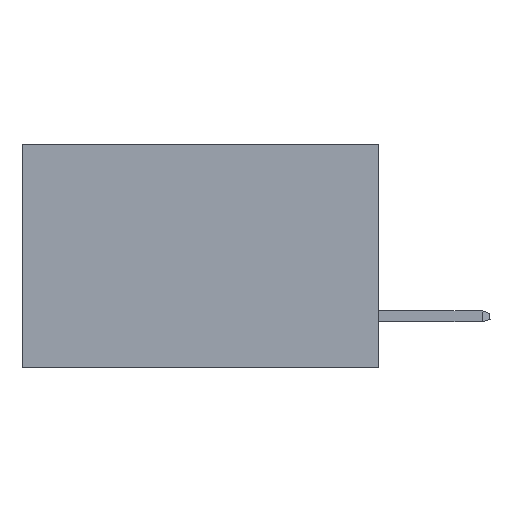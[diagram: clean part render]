
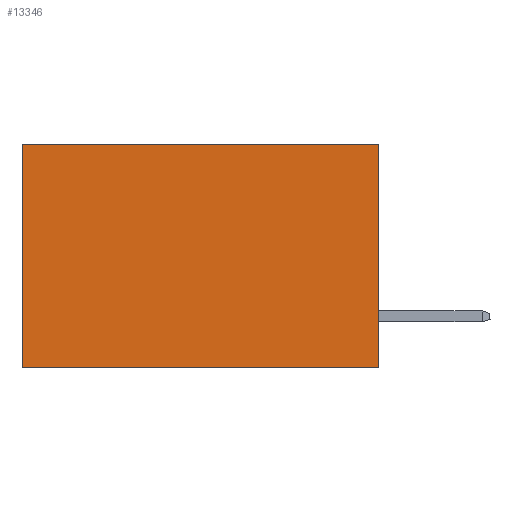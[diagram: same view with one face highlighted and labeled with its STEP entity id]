
A CAD part, left-side view. The second image highlights one B-rep face of the part: STEP entity #13346.
In plain terms, the highlighted planar face has unit normal (-1, 0, 0).
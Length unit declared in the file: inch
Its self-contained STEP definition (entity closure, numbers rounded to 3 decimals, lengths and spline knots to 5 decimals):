
#583 = CARTESIAN_POINT ( 'NONE',  ( 0.277, 0.59, 0. ) ) ;
#1040 = CARTESIAN_POINT ( 'NONE',  ( 0.277, 0.59, -0.37 ) ) ;
#2167 = CARTESIAN_POINT ( 'NONE',  ( 0.277, 0., -0.37 ) ) ;
#2836 = ORIENTED_EDGE ( 'NONE', *, *, #13475, .F. ) ;
#3219 = DIRECTION ( 'NONE',  ( 0., 0., -1. ) ) ;
#3410 = DIRECTION ( 'NONE',  ( 0., 0., -1. ) ) ;
#3640 = VERTEX_POINT ( 'NONE', #583 ) ;
#4572 = LINE ( 'NONE', #5837, #11000 ) ;
#4634 = DIRECTION ( 'NONE',  ( 0., 0., -1. ) ) ;
#5372 = VECTOR ( 'NONE', #3219, 39.37008 ) ;
#5837 = CARTESIAN_POINT ( 'NONE',  ( 0.277, 0.59, -0.37 ) ) ;
#6148 = LINE ( 'NONE', #15330, #5372 ) ;
#8121 = EDGE_LOOP ( 'NONE', ( #24821, #2836, #28118, #8788 ) ) ;
#8788 = ORIENTED_EDGE ( 'NONE', *, *, #18326, .T. ) ;
#9919 = CARTESIAN_POINT ( 'NONE',  ( 0.277, 0., -0.37 ) ) ;
#11000 = VECTOR ( 'NONE', #3410, 39.37008 ) ;
#11846 = VERTEX_POINT ( 'NONE', #1040 ) ;
#11935 = CARTESIAN_POINT ( 'NONE',  ( 0.277, 0., 0. ) ) ;
#13346 = ADVANCED_FACE ( 'NONE', ( #30625 ), #28491, .F. ) ;
#13475 = EDGE_CURVE ( 'NONE', #28174, #11846, #15902, .T. ) ;
#13645 = AXIS2_PLACEMENT_3D ( 'NONE', #2167, #19214, #4634 ) ;
#13772 = LINE ( 'NONE', #11935, #20226 ) ;
#15112 = VECTOR ( 'NONE', #29013, 39.37008 ) ;
#15330 = CARTESIAN_POINT ( 'NONE',  ( 0.277, 0., -0.37 ) ) ;
#15902 = LINE ( 'NONE', #9919, #15112 ) ;
#18326 = EDGE_CURVE ( 'NONE', #23925, #3640, #13772, .T. ) ;
#18564 = EDGE_CURVE ( 'NONE', #23925, #28174, #6148, .T. ) ;
#19057 = CARTESIAN_POINT ( 'NONE',  ( 0.277, 0., -0.37 ) ) ;
#19214 = DIRECTION ( 'NONE',  ( 1., 0., 0. ) ) ;
#20128 = CARTESIAN_POINT ( 'NONE',  ( 0.277, 0., 0. ) ) ;
#20226 = VECTOR ( 'NONE', #26206, 39.37008 ) ;
#23925 = VERTEX_POINT ( 'NONE', #20128 ) ;
#24821 = ORIENTED_EDGE ( 'NONE', *, *, #30432, .T. ) ;
#26206 = DIRECTION ( 'NONE',  ( 0., 1., 0. ) ) ;
#28118 = ORIENTED_EDGE ( 'NONE', *, *, #18564, .F. ) ;
#28174 = VERTEX_POINT ( 'NONE', #19057 ) ;
#28491 = PLANE ( 'NONE',  #13645 ) ;
#29013 = DIRECTION ( 'NONE',  ( 0., 1., 0. ) ) ;
#30432 = EDGE_CURVE ( 'NONE', #3640, #11846, #4572, .T. ) ;
#30625 = FACE_OUTER_BOUND ( 'NONE', #8121, .T. ) ;
